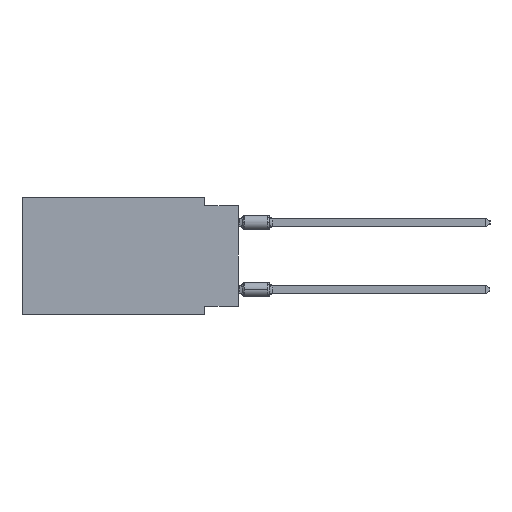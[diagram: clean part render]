
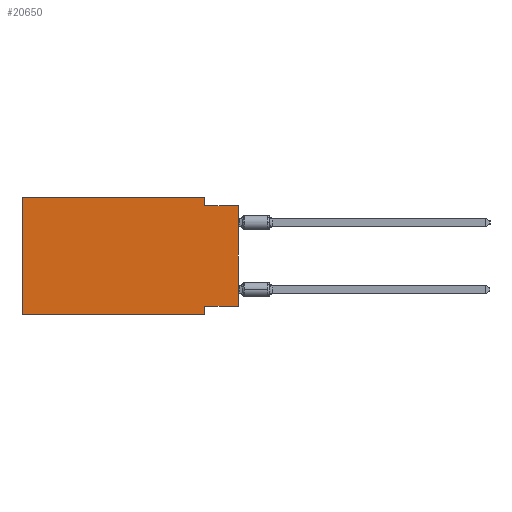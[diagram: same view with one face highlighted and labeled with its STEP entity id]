
A CAD part, left-side view. The second image highlights one B-rep face of the part: STEP entity #20650.
In plain terms, the highlighted planar face has unit normal (-1, 0, 0).
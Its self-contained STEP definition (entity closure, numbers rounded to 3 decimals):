
#52 = FACE_OUTER_BOUND ( 'NONE', #21206, .T. ) ;
#225 = LINE ( 'NONE', #23758, #17866 ) ;
#356 = AXIS2_PLACEMENT_3D ( 'NONE', #5822, #28897, #4919 ) ;
#981 = EDGE_CURVE ( 'NONE', #21164, #2984, #19157, .T. ) ;
#1477 = ORIENTED_EDGE ( 'NONE', *, *, #11939, .T. ) ;
#1627 = VECTOR ( 'NONE', #28705, 1000. ) ;
#1837 = LINE ( 'NONE', #24224, #7906 ) ;
#2845 = ORIENTED_EDGE ( 'NONE', *, *, #981, .F. ) ;
#2948 = VECTOR ( 'NONE', #8627, 1000. ) ;
#2984 = VERTEX_POINT ( 'NONE', #6797 ) ;
#4608 = VERTEX_POINT ( 'NONE', #11446 ) ;
#4919 = DIRECTION ( 'NONE',  ( 0., 0., -1. ) ) ;
#4977 = LINE ( 'NONE', #16741, #8753 ) ;
#5419 = DIRECTION ( 'NONE',  ( 0., 1., 0. ) ) ;
#5487 = VECTOR ( 'NONE', #20452, 1000. ) ;
#5822 = CARTESIAN_POINT ( 'NONE',  ( 0., 16.383, 0. ) ) ;
#5895 = CARTESIAN_POINT ( 'NONE',  ( 0., 0., -8.255 ) ) ;
#6326 = EDGE_CURVE ( 'NONE', #17497, #21164, #4977, .T. ) ;
#6356 = DIRECTION ( 'NONE',  ( 0., -1., 0. ) ) ;
#6797 = CARTESIAN_POINT ( 'NONE',  ( 0., 2.54, 0. ) ) ;
#7364 = EDGE_CURVE ( 'NONE', #21267, #4608, #225, .T. ) ;
#7906 = VECTOR ( 'NONE', #21727, 1000. ) ;
#8627 = DIRECTION ( 'NONE',  ( 0., 0., 1. ) ) ;
#8753 = VECTOR ( 'NONE', #19102, 1000. ) ;
#10880 = CARTESIAN_POINT ( 'NONE',  ( 0., 2.54, 0. ) ) ;
#11446 = CARTESIAN_POINT ( 'NONE',  ( 0., 0., -0.635 ) ) ;
#11567 = CARTESIAN_POINT ( 'NONE',  ( 0., 2.54, -0.635 ) ) ;
#11939 = EDGE_CURVE ( 'NONE', #17497, #24233, #27354, .T. ) ;
#12448 = CARTESIAN_POINT ( 'NONE',  ( 0., 16.383, -8.89 ) ) ;
#12738 = VECTOR ( 'NONE', #6356, 1000. ) ;
#13308 = CARTESIAN_POINT ( 'NONE',  ( 0., 16.383, 0. ) ) ;
#14404 = EDGE_CURVE ( 'NONE', #19135, #25896, #15440, .T. ) ;
#15440 = LINE ( 'NONE', #5895, #22573 ) ;
#16129 = ORIENTED_EDGE ( 'NONE', *, *, #21970, .F. ) ;
#16741 = CARTESIAN_POINT ( 'NONE',  ( 0., 16.383, 0. ) ) ;
#17497 = VERTEX_POINT ( 'NONE', #12448 ) ;
#17866 = VECTOR ( 'NONE', #23905, 1000. ) ;
#18647 = EDGE_CURVE ( 'NONE', #19135, #4608, #18912, .T. ) ;
#18912 = LINE ( 'NONE', #30093, #2948 ) ;
#19027 = CARTESIAN_POINT ( 'NONE',  ( 0., 0., -8.255 ) ) ;
#19102 = DIRECTION ( 'NONE',  ( 0., 0., 1. ) ) ;
#19135 = VERTEX_POINT ( 'NONE', #19027 ) ;
#19157 = LINE ( 'NONE', #24160, #1627 ) ;
#19198 = PLANE ( 'NONE',  #356 ) ;
#19584 = ORIENTED_EDGE ( 'NONE', *, *, #23989, .F. ) ;
#20234 = ORIENTED_EDGE ( 'NONE', *, *, #18647, .T. ) ;
#20452 = DIRECTION ( 'NONE',  ( 0., 0., -1. ) ) ;
#20650 = ADVANCED_FACE ( 'NONE', ( #52 ), #19198, .F. ) ;
#21164 = VERTEX_POINT ( 'NONE', #13308 ) ;
#21206 = EDGE_LOOP ( 'NONE', ( #20234, #26163, #16129, #2845, #24267, #1477, #19584, #27449 ) ) ;
#21267 = VERTEX_POINT ( 'NONE', #11567 ) ;
#21727 = DIRECTION ( 'NONE',  ( 0., 0., -1. ) ) ;
#21970 = EDGE_CURVE ( 'NONE', #2984, #21267, #24671, .T. ) ;
#22573 = VECTOR ( 'NONE', #5419, 1000. ) ;
#23758 = CARTESIAN_POINT ( 'NONE',  ( 0., 0., -0.635 ) ) ;
#23905 = DIRECTION ( 'NONE',  ( 0., -1., 0. ) ) ;
#23989 = EDGE_CURVE ( 'NONE', #25896, #24233, #1837, .T. ) ;
#24160 = CARTESIAN_POINT ( 'NONE',  ( 0., 16.383, 0. ) ) ;
#24224 = CARTESIAN_POINT ( 'NONE',  ( 0., 2.54, -8.89 ) ) ;
#24233 = VERTEX_POINT ( 'NONE', #25625 ) ;
#24267 = ORIENTED_EDGE ( 'NONE', *, *, #6326, .F. ) ;
#24671 = LINE ( 'NONE', #10880, #5487 ) ;
#25625 = CARTESIAN_POINT ( 'NONE',  ( 0., 2.54, -8.89 ) ) ;
#25892 = CARTESIAN_POINT ( 'NONE',  ( 0., 2.54, -8.255 ) ) ;
#25896 = VERTEX_POINT ( 'NONE', #25892 ) ;
#26163 = ORIENTED_EDGE ( 'NONE', *, *, #7364, .F. ) ;
#27354 = LINE ( 'NONE', #27821, #12738 ) ;
#27449 = ORIENTED_EDGE ( 'NONE', *, *, #14404, .F. ) ;
#27821 = CARTESIAN_POINT ( 'NONE',  ( 0., 16.383, -8.89 ) ) ;
#28705 = DIRECTION ( 'NONE',  ( 0., -1., 0. ) ) ;
#28897 = DIRECTION ( 'NONE',  ( 1., 0., 0. ) ) ;
#30093 = CARTESIAN_POINT ( 'NONE',  ( 0., 0., 0. ) ) ;
